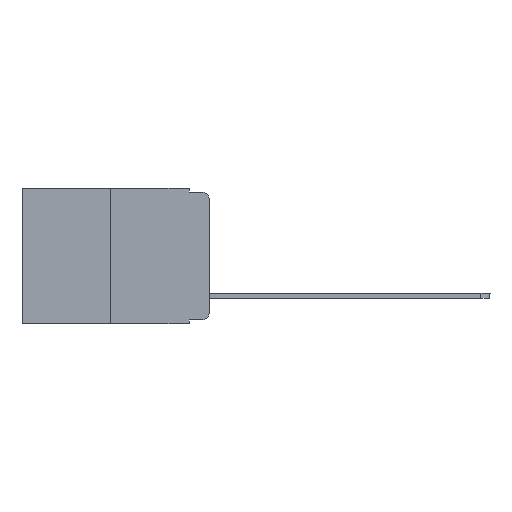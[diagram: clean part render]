
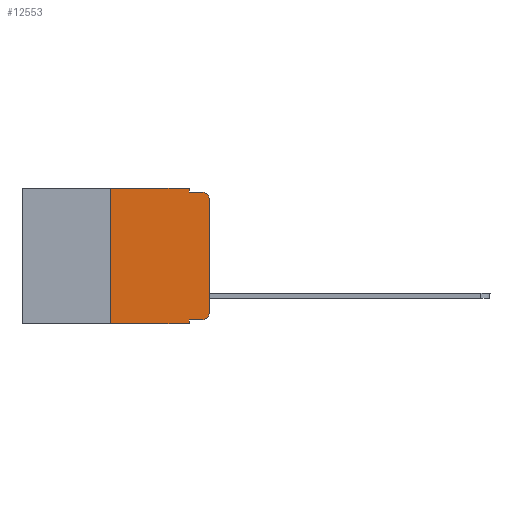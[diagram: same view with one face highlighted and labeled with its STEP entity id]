
A CAD part, left-side view. The second image highlights one B-rep face of the part: STEP entity #12553.
In plain terms, the highlighted planar face has unit normal (-1, 0, 0).
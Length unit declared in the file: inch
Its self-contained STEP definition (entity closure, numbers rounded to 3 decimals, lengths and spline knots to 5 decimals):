
#22 = CARTESIAN_POINT ( 'NONE',  ( 0., 0., -0.313 ) ) ;
#24 = CARTESIAN_POINT ( 'NONE',  ( 0., 0.051, -0.01 ) ) ;
#236 = EDGE_CURVE ( 'NONE', #7609, #3248, #11186, .T. ) ;
#341 = LINE ( 'NONE', #8017, #15344 ) ;
#427 = DIRECTION ( 'NONE',  ( 0., 0., -1. ) ) ;
#479 = VERTEX_POINT ( 'NONE', #15642 ) ;
#686 = ORIENTED_EDGE ( 'NONE', *, *, #236, .F. ) ;
#1100 = DIRECTION ( 'NONE',  ( -1., 0., 0. ) ) ;
#1145 = VERTEX_POINT ( 'NONE', #22 ) ;
#1494 = DIRECTION ( 'NONE',  ( 0., -1., 0. ) ) ;
#1519 = ORIENTED_EDGE ( 'NONE', *, *, #15570, .T. ) ;
#3039 = CIRCLE ( 'NONE', #16452, 0.02 ) ;
#3129 = ORIENTED_EDGE ( 'NONE', *, *, #9687, .F. ) ;
#3248 = VERTEX_POINT ( 'NONE', #12375 ) ;
#3263 = ORIENTED_EDGE ( 'NONE', *, *, #4825, .T. ) ;
#3911 = DIRECTION ( 'NONE',  ( 0., -1., 0. ) ) ;
#4110 = LINE ( 'NONE', #5249, #7685 ) ;
#4138 = CARTESIAN_POINT ( 'NONE',  ( 0., 0.473, -0.343 ) ) ;
#4203 = CARTESIAN_POINT ( 'NONE',  ( 0., 0.473, 0. ) ) ;
#4295 = VECTOR ( 'NONE', #15217, 39.37008 ) ;
#4454 = VERTEX_POINT ( 'NONE', #7645 ) ;
#4717 = CARTESIAN_POINT ( 'NONE',  ( 0., 0., -0.03 ) ) ;
#4825 = EDGE_CURVE ( 'NONE', #9301, #4454, #16130, .T. ) ;
#4983 = ORIENTED_EDGE ( 'NONE', *, *, #6338, .T. ) ;
#5079 = AXIS2_PLACEMENT_3D ( 'NONE', #11823, #1100, #5429 ) ;
#5249 = CARTESIAN_POINT ( 'NONE',  ( 0., 0., 0. ) ) ;
#5332 = PLANE ( 'NONE',  #16574 ) ;
#5429 = DIRECTION ( 'NONE',  ( 0., 0., -1. ) ) ;
#5444 = ORIENTED_EDGE ( 'NONE', *, *, #11897, .T. ) ;
#5476 = CARTESIAN_POINT ( 'NONE',  ( 0., 0.051, 0. ) ) ;
#5490 = ORIENTED_EDGE ( 'NONE', *, *, #10009, .F. ) ;
#5571 = CARTESIAN_POINT ( 'NONE',  ( 0., 0.25, -0.343 ) ) ;
#6321 = LINE ( 'NONE', #13049, #8239 ) ;
#6338 = EDGE_CURVE ( 'NONE', #479, #1145, #14586, .T. ) ;
#6827 = VERTEX_POINT ( 'NONE', #13022 ) ;
#6999 = DIRECTION ( 'NONE',  ( 0., 0., -1. ) ) ;
#7609 = VERTEX_POINT ( 'NONE', #24 ) ;
#7645 = CARTESIAN_POINT ( 'NONE',  ( 0., 0.051, -0.343 ) ) ;
#7685 = VECTOR ( 'NONE', #15939, 39.37008 ) ;
#8017 = CARTESIAN_POINT ( 'NONE',  ( 0., 0.051, 0. ) ) ;
#8239 = VECTOR ( 'NONE', #17107, 39.37008 ) ;
#8745 = VERTEX_POINT ( 'NONE', #15709 ) ;
#8979 = CARTESIAN_POINT ( 'NONE',  ( 0., 0.473, 0. ) ) ;
#9300 = EDGE_CURVE ( 'NONE', #8745, #4454, #9330, .T. ) ;
#9301 = VERTEX_POINT ( 'NONE', #5571 ) ;
#9330 = LINE ( 'NONE', #5476, #10965 ) ;
#9365 = EDGE_CURVE ( 'NONE', #8745, #479, #14769, .T. ) ;
#9454 = EDGE_LOOP ( 'NONE', ( #5444, #1519, #686, #10379, #3129, #5490, #3263, #11793, #14282, #4983 ) ) ;
#9508 = DIRECTION ( 'NONE',  ( 0., 0., -1. ) ) ;
#9687 = EDGE_CURVE ( 'NONE', #13568, #6827, #15651, .T. ) ;
#10009 = EDGE_CURVE ( 'NONE', #9301, #13568, #6321, .T. ) ;
#10379 = ORIENTED_EDGE ( 'NONE', *, *, #15487, .F. ) ;
#10764 = FACE_OUTER_BOUND ( 'NONE', #9454, .T. ) ;
#10965 = VECTOR ( 'NONE', #9508, 39.37008 ) ;
#11186 = LINE ( 'NONE', #16524, #4295 ) ;
#11793 = ORIENTED_EDGE ( 'NONE', *, *, #9300, .F. ) ;
#11823 = CARTESIAN_POINT ( 'NONE',  ( 0., 0.02, -0.313 ) ) ;
#11897 = EDGE_CURVE ( 'NONE', #1145, #12707, #4110, .T. ) ;
#12375 = CARTESIAN_POINT ( 'NONE',  ( 0., 0.02, -0.01 ) ) ;
#12553 = ADVANCED_FACE ( 'NONE', ( #10764 ), #5332, .F. ) ;
#12688 = VECTOR ( 'NONE', #3911, 39.37008 ) ;
#12707 = VERTEX_POINT ( 'NONE', #4717 ) ;
#13022 = CARTESIAN_POINT ( 'NONE',  ( 0., 0.051, 0. ) ) ;
#13049 = CARTESIAN_POINT ( 'NONE',  ( 0., 0.25, 0. ) ) ;
#13448 = CARTESIAN_POINT ( 'NONE',  ( 0., 0.051, -0.333 ) ) ;
#13568 = VERTEX_POINT ( 'NONE', #16913 ) ;
#13765 = DIRECTION ( 'NONE',  ( 0., -1., 0. ) ) ;
#14142 = CARTESIAN_POINT ( 'NONE',  ( 0., 0.02, -0.03 ) ) ;
#14282 = ORIENTED_EDGE ( 'NONE', *, *, #9365, .T. ) ;
#14586 = CIRCLE ( 'NONE', #5079, 0.02 ) ;
#14769 = LINE ( 'NONE', #13448, #16862 ) ;
#14833 = VECTOR ( 'NONE', #13765, 39.37008 ) ;
#15217 = DIRECTION ( 'NONE',  ( 0., -1., 0. ) ) ;
#15229 = DIRECTION ( 'NONE',  ( -1., 0., 0. ) ) ;
#15344 = VECTOR ( 'NONE', #427, 39.37008 ) ;
#15412 = DIRECTION ( 'NONE',  ( 0., 0., -1. ) ) ;
#15487 = EDGE_CURVE ( 'NONE', #6827, #7609, #341, .T. ) ;
#15570 = EDGE_CURVE ( 'NONE', #12707, #3248, #3039, .T. ) ;
#15642 = CARTESIAN_POINT ( 'NONE',  ( 0., 0.02, -0.333 ) ) ;
#15651 = LINE ( 'NONE', #8979, #12688 ) ;
#15709 = CARTESIAN_POINT ( 'NONE',  ( 0., 0.051, -0.333 ) ) ;
#15939 = DIRECTION ( 'NONE',  ( 0., 0., 1. ) ) ;
#16096 = DIRECTION ( 'NONE',  ( 1., 0., 0. ) ) ;
#16130 = LINE ( 'NONE', #4138, #14833 ) ;
#16452 = AXIS2_PLACEMENT_3D ( 'NONE', #14142, #15229, #15412 ) ;
#16524 = CARTESIAN_POINT ( 'NONE',  ( 0., 0.051, -0.01 ) ) ;
#16574 = AXIS2_PLACEMENT_3D ( 'NONE', #4203, #16096, #6999 ) ;
#16862 = VECTOR ( 'NONE', #1494, 39.37008 ) ;
#16913 = CARTESIAN_POINT ( 'NONE',  ( 0., 0.25, 0. ) ) ;
#17107 = DIRECTION ( 'NONE',  ( 0., 0., 1. ) ) ;
